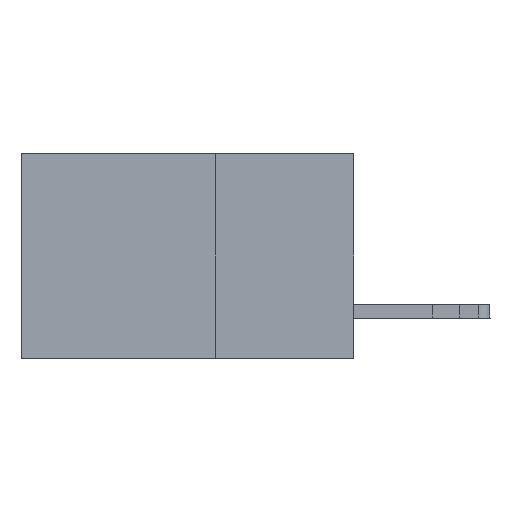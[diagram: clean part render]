
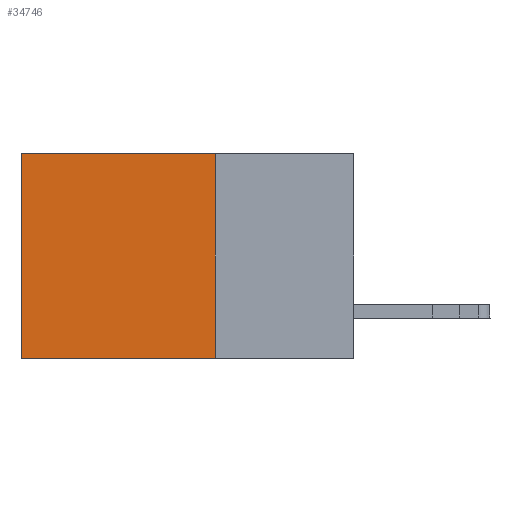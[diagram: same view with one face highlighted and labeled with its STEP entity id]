
A CAD part, left-side view. The second image highlights one B-rep face of the part: STEP entity #34746.
In plain terms, the highlighted planar face has unit normal (-1, 0, 0).
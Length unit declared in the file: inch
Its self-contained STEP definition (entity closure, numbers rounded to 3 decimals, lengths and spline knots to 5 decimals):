
#1251 = DIRECTION ( 'NONE',  ( 0., 0., -1. ) ) ;
#2413 = CARTESIAN_POINT ( 'NONE',  ( 0.2875, 0.25, 0. ) ) ;
#2559 = CARTESIAN_POINT ( 'NONE',  ( 0.2875, 0.6, 0. ) ) ;
#3148 = ORIENTED_EDGE ( 'NONE', *, *, #14089, .F. ) ;
#4951 = ORIENTED_EDGE ( 'NONE', *, *, #29431, .T. ) ;
#5030 = VERTEX_POINT ( 'NONE', #21854 ) ;
#6991 = CARTESIAN_POINT ( 'NONE',  ( 0.2875, 0.25, 0. ) ) ;
#7617 = CARTESIAN_POINT ( 'NONE',  ( 0.2875, 0.25, 0. ) ) ;
#8153 = PLANE ( 'NONE',  #11747 ) ;
#10842 = VERTEX_POINT ( 'NONE', #6991 ) ;
#10934 = ORIENTED_EDGE ( 'NONE', *, *, #20413, .T. ) ;
#11019 = DIRECTION ( 'NONE',  ( 0., 0., -1. ) ) ;
#11747 = AXIS2_PLACEMENT_3D ( 'NONE', #2413, #28195, #11019 ) ;
#13782 = EDGE_LOOP ( 'NONE', ( #10934, #28458, #3148, #4951 ) ) ;
#13821 = VECTOR ( 'NONE', #33399, 39.37008 ) ;
#14089 = EDGE_CURVE ( 'NONE', #10842, #5030, #30401, .T. ) ;
#16255 = DIRECTION ( 'NONE',  ( 0., 1., 0. ) ) ;
#16655 = FACE_OUTER_BOUND ( 'NONE', #13782, .T. ) ;
#20413 = EDGE_CURVE ( 'NONE', #31921, #35888, #33189, .T. ) ;
#21488 = LINE ( 'NONE', #30528, #13821 ) ;
#21854 = CARTESIAN_POINT ( 'NONE',  ( 0.2875, 0.25, -0.37 ) ) ;
#22757 = VECTOR ( 'NONE', #32956, 39.37008 ) ;
#24166 = CARTESIAN_POINT ( 'NONE',  ( 0.2875, 0.6, 0. ) ) ;
#28185 = LINE ( 'NONE', #7617, #34886 ) ;
#28195 = DIRECTION ( 'NONE',  ( 1., 0., 0. ) ) ;
#28458 = ORIENTED_EDGE ( 'NONE', *, *, #29420, .F. ) ;
#29420 = EDGE_CURVE ( 'NONE', #5030, #35888, #21488, .T. ) ;
#29431 = EDGE_CURVE ( 'NONE', #10842, #31921, #28185, .T. ) ;
#30067 = CARTESIAN_POINT ( 'NONE',  ( 0.2875, 0.25, 0. ) ) ;
#30401 = LINE ( 'NONE', #30067, #22757 ) ;
#30528 = CARTESIAN_POINT ( 'NONE',  ( 0.2875, 0.25, -0.37 ) ) ;
#31921 = VERTEX_POINT ( 'NONE', #2559 ) ;
#32298 = VECTOR ( 'NONE', #1251, 39.37008 ) ;
#32956 = DIRECTION ( 'NONE',  ( 0., 0., -1. ) ) ;
#33189 = LINE ( 'NONE', #24166, #32298 ) ;
#33399 = DIRECTION ( 'NONE',  ( 0., 1., 0. ) ) ;
#33879 = CARTESIAN_POINT ( 'NONE',  ( 0.2875, 0.6, -0.37 ) ) ;
#34746 = ADVANCED_FACE ( 'NONE', ( #16655 ), #8153, .F. ) ;
#34886 = VECTOR ( 'NONE', #16255, 39.37008 ) ;
#35888 = VERTEX_POINT ( 'NONE', #33879 ) ;
